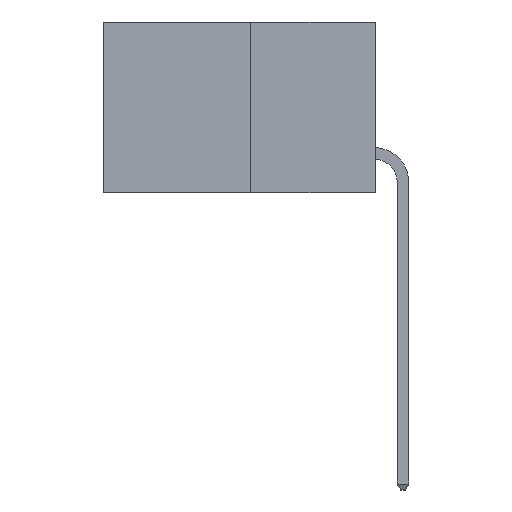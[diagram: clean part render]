
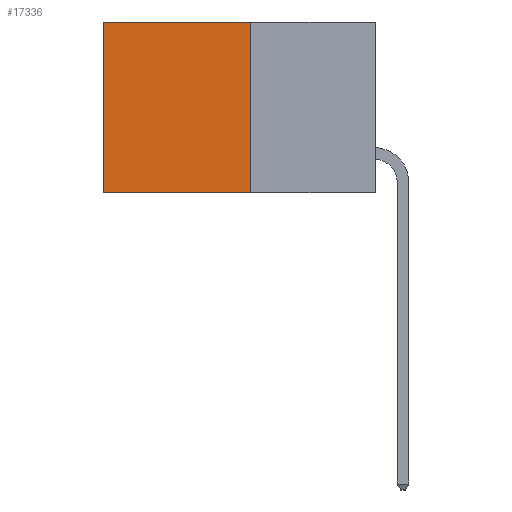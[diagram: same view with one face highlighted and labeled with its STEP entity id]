
A CAD part, left-side view. The second image highlights one B-rep face of the part: STEP entity #17336.
In plain terms, the highlighted planar face has unit normal (-1, 0, 0).
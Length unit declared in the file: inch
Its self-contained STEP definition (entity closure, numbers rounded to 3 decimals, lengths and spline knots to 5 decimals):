
#538 = ORIENTED_EDGE ( 'NONE', *, *, #4900, .F. ) ;
#605 = PLANE ( 'NONE',  #16189 ) ;
#667 = DIRECTION ( 'NONE',  ( 1., 0., 0. ) ) ;
#2046 = VECTOR ( 'NONE', #7039, 39.37008 ) ;
#2749 = LINE ( 'NONE', #7874, #16924 ) ;
#2970 = CARTESIAN_POINT ( 'NONE',  ( 0.277, 0.59, -0.37 ) ) ;
#3551 = LINE ( 'NONE', #2970, #10457 ) ;
#4900 = EDGE_CURVE ( 'NONE', #16214, #6142, #6027, .T. ) ;
#5835 = LINE ( 'NONE', #9742, #2046 ) ;
#6027 = LINE ( 'NONE', #6761, #16877 ) ;
#6142 = VERTEX_POINT ( 'NONE', #9994 ) ;
#6761 = CARTESIAN_POINT ( 'NONE',  ( 0.277, 0.27, -0.37 ) ) ;
#6888 = DIRECTION ( 'NONE',  ( 0., 1., 0. ) ) ;
#7039 = DIRECTION ( 'NONE',  ( 0., 0., -1. ) ) ;
#7874 = CARTESIAN_POINT ( 'NONE',  ( 0.277, 0.27, 0. ) ) ;
#8505 = ORIENTED_EDGE ( 'NONE', *, *, #13418, .F. ) ;
#8572 = CARTESIAN_POINT ( 'NONE',  ( 0.277, 0.27, 0. ) ) ;
#9141 = CARTESIAN_POINT ( 'NONE',  ( 0.277, 0.27, -0.37 ) ) ;
#9548 = VERTEX_POINT ( 'NONE', #14065 ) ;
#9742 = CARTESIAN_POINT ( 'NONE',  ( 0.277, 0.27, -0.37 ) ) ;
#9841 = EDGE_LOOP ( 'NONE', ( #11321, #538, #8505, #12165 ) ) ;
#9994 = CARTESIAN_POINT ( 'NONE',  ( 0.277, 0.59, -0.37 ) ) ;
#10188 = EDGE_CURVE ( 'NONE', #9548, #6142, #3551, .T. ) ;
#10457 = VECTOR ( 'NONE', #11276, 39.37008 ) ;
#10511 = DIRECTION ( 'NONE',  ( 0., 0., -1. ) ) ;
#10865 = CARTESIAN_POINT ( 'NONE',  ( 0.277, 0.27, -0.37 ) ) ;
#11276 = DIRECTION ( 'NONE',  ( 0., 0., -1. ) ) ;
#11321 = ORIENTED_EDGE ( 'NONE', *, *, #10188, .T. ) ;
#11592 = VERTEX_POINT ( 'NONE', #8572 ) ;
#12165 = ORIENTED_EDGE ( 'NONE', *, *, #13162, .T. ) ;
#12992 = FACE_OUTER_BOUND ( 'NONE', #9841, .T. ) ;
#13162 = EDGE_CURVE ( 'NONE', #11592, #9548, #2749, .T. ) ;
#13409 = DIRECTION ( 'NONE',  ( 0., 1., 0. ) ) ;
#13418 = EDGE_CURVE ( 'NONE', #11592, #16214, #5835, .T. ) ;
#14065 = CARTESIAN_POINT ( 'NONE',  ( 0.277, 0.59, 0. ) ) ;
#16189 = AXIS2_PLACEMENT_3D ( 'NONE', #9141, #667, #10511 ) ;
#16214 = VERTEX_POINT ( 'NONE', #10865 ) ;
#16877 = VECTOR ( 'NONE', #6888, 39.37008 ) ;
#16924 = VECTOR ( 'NONE', #13409, 39.37008 ) ;
#17336 = ADVANCED_FACE ( 'NONE', ( #12992 ), #605, .F. ) ;
